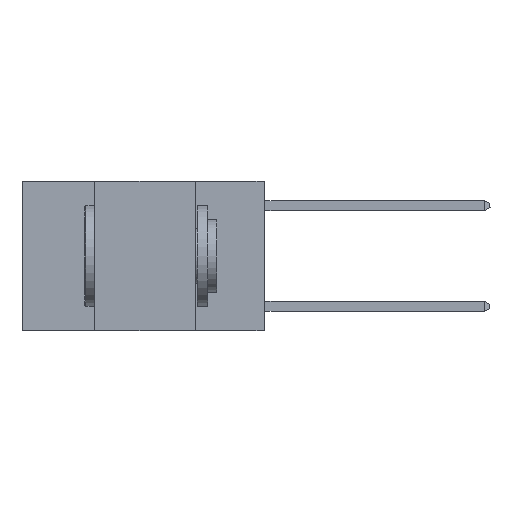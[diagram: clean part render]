
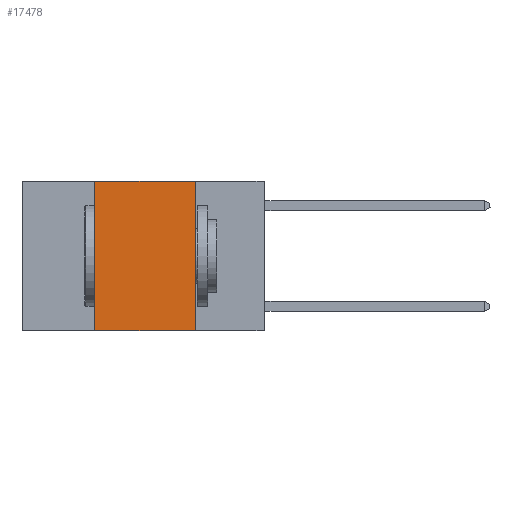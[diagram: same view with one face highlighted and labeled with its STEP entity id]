
A CAD part, left-side view. The second image highlights one B-rep face of the part: STEP entity #17478.
In plain terms, the highlighted planar face has unit normal (-1, 0, 0).
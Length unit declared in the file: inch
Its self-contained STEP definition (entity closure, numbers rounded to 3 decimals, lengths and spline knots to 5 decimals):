
#163 = CARTESIAN_POINT ( 'NONE',  ( 0., 0.6, 0. ) ) ;
#1087 = EDGE_CURVE ( 'NONE', #5662, #10558, #7801, .T. ) ;
#1336 = CARTESIAN_POINT ( 'NONE',  ( 0., 0.17, -0.37 ) ) ;
#1692 = VERTEX_POINT ( 'NONE', #17235 ) ;
#2024 = DIRECTION ( 'NONE',  ( 0., 0., -1. ) ) ;
#2619 = ORIENTED_EDGE ( 'NONE', *, *, #15182, .F. ) ;
#2700 = EDGE_CURVE ( 'NONE', #1692, #11516, #12989, .T. ) ;
#2732 = EDGE_LOOP ( 'NONE', ( #11013, #13566, #2619, #5804 ) ) ;
#3057 = VECTOR ( 'NONE', #16911, 39.37008 ) ;
#3827 = CARTESIAN_POINT ( 'NONE',  ( 0., 0.42, 0. ) ) ;
#4175 = CARTESIAN_POINT ( 'NONE',  ( 0., 0.42, -0.37 ) ) ;
#4927 = EDGE_CURVE ( 'NONE', #11516, #10558, #10302, .T. ) ;
#5397 = VECTOR ( 'NONE', #18970, 39.37008 ) ;
#5662 = VERTEX_POINT ( 'NONE', #4175 ) ;
#5753 = LINE ( 'NONE', #3827, #10674 ) ;
#5804 = ORIENTED_EDGE ( 'NONE', *, *, #1087, .T. ) ;
#5856 = AXIS2_PLACEMENT_3D ( 'NONE', #163, #13196, #2024 ) ;
#7801 = LINE ( 'NONE', #11668, #17151 ) ;
#10302 = LINE ( 'NONE', #13321, #5397 ) ;
#10558 = VERTEX_POINT ( 'NONE', #1336 ) ;
#10674 = VECTOR ( 'NONE', #16885, 39.37008 ) ;
#11013 = ORIENTED_EDGE ( 'NONE', *, *, #4927, .F. ) ;
#11516 = VERTEX_POINT ( 'NONE', #15149 ) ;
#11600 = DIRECTION ( 'NONE',  ( 0., -1., 0. ) ) ;
#11668 = CARTESIAN_POINT ( 'NONE',  ( 0., 0.6, -0.37 ) ) ;
#12989 = LINE ( 'NONE', #17679, #3057 ) ;
#13196 = DIRECTION ( 'NONE',  ( 1., 0., 0. ) ) ;
#13321 = CARTESIAN_POINT ( 'NONE',  ( 0., 0.17, 0. ) ) ;
#13566 = ORIENTED_EDGE ( 'NONE', *, *, #2700, .F. ) ;
#15149 = CARTESIAN_POINT ( 'NONE',  ( 0., 0.17, 0. ) ) ;
#15182 = EDGE_CURVE ( 'NONE', #5662, #1692, #5753, .T. ) ;
#16885 = DIRECTION ( 'NONE',  ( 0., 0., 1. ) ) ;
#16911 = DIRECTION ( 'NONE',  ( 0., -1., 0. ) ) ;
#17151 = VECTOR ( 'NONE', #11600, 39.37008 ) ;
#17235 = CARTESIAN_POINT ( 'NONE',  ( 0., 0.42, 0. ) ) ;
#17478 = ADVANCED_FACE ( 'NONE', ( #18217 ), #20621, .F. ) ;
#17679 = CARTESIAN_POINT ( 'NONE',  ( 0., 0.6, 0. ) ) ;
#18217 = FACE_OUTER_BOUND ( 'NONE', #2732, .T. ) ;
#18970 = DIRECTION ( 'NONE',  ( 0., 0., -1. ) ) ;
#20621 = PLANE ( 'NONE',  #5856 ) ;
